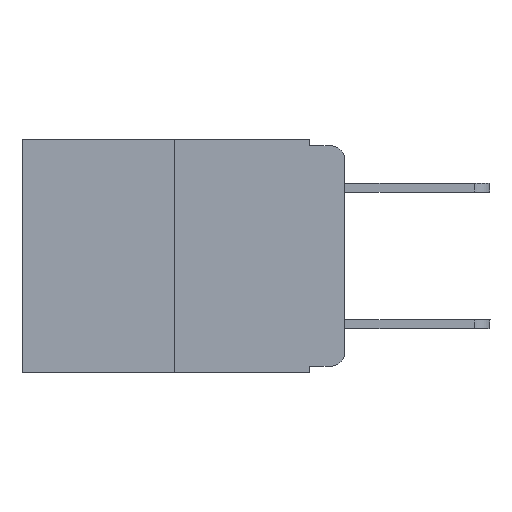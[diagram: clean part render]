
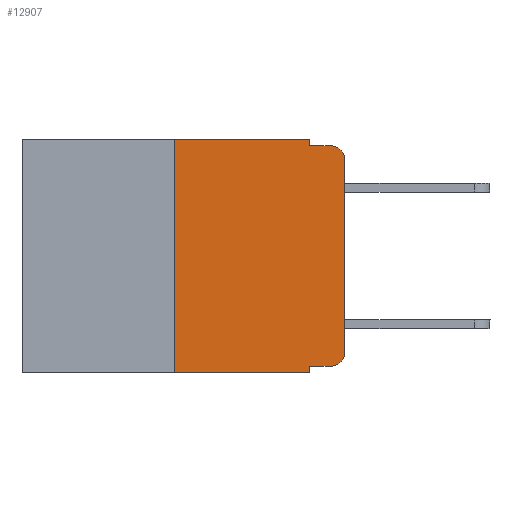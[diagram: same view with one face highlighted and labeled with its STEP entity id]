
A CAD part, left-side view. The second image highlights one B-rep face of the part: STEP entity #12907.
In plain terms, the highlighted planar face has unit normal (-1, 0, 0).
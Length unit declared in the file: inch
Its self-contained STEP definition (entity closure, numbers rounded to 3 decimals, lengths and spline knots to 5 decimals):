
#98 = AXIS2_PLACEMENT_3D ( 'NONE', #14509, #1699, #7501 ) ;
#139 = CARTESIAN_POINT ( 'NONE',  ( 0., 0.25, 0. ) ) ;
#285 = ORIENTED_EDGE ( 'NONE', *, *, #360, .T. ) ;
#360 = EDGE_CURVE ( 'NONE', #15100, #4920, #1604, .T. ) ;
#596 = VERTEX_POINT ( 'NONE', #11716 ) ;
#723 = CARTESIAN_POINT ( 'NONE',  ( 0., 0.051, -0.01 ) ) ;
#1584 = AXIS2_PLACEMENT_3D ( 'NONE', #2844, #2794, #10892 ) ;
#1585 = DIRECTION ( 'NONE',  ( 0., -1., 0. ) ) ;
#1597 = ORIENTED_EDGE ( 'NONE', *, *, #11966, .T. ) ;
#1604 = CIRCLE ( 'NONE', #98, 0.02 ) ;
#1699 = DIRECTION ( 'NONE',  ( -1., 0., 0. ) ) ;
#1790 = LINE ( 'NONE', #139, #7619 ) ;
#2120 = EDGE_CURVE ( 'NONE', #596, #11708, #8279, .T. ) ;
#2179 = CARTESIAN_POINT ( 'NONE',  ( 0., 0.051, 0. ) ) ;
#2493 = DIRECTION ( 'NONE',  ( 0., 0., 1. ) ) ;
#2783 = CARTESIAN_POINT ( 'NONE',  ( 0., 0.25, -0.343 ) ) ;
#2794 = DIRECTION ( 'NONE',  ( 1., 0., 0. ) ) ;
#2844 = CARTESIAN_POINT ( 'NONE',  ( 0., 0.473, 0. ) ) ;
#3056 = CARTESIAN_POINT ( 'NONE',  ( 0., 0.051, 0. ) ) ;
#3266 = VECTOR ( 'NONE', #13097, 39.37008 ) ;
#3449 = ORIENTED_EDGE ( 'NONE', *, *, #2120, .T. ) ;
#4105 = VECTOR ( 'NONE', #1585, 39.37008 ) ;
#4127 = DIRECTION ( 'NONE',  ( 0., -1., 0. ) ) ;
#4250 = VERTEX_POINT ( 'NONE', #3056 ) ;
#4324 = CARTESIAN_POINT ( 'NONE',  ( 0., 0.051, -0.01 ) ) ;
#4416 = ORIENTED_EDGE ( 'NONE', *, *, #10406, .F. ) ;
#4563 = CIRCLE ( 'NONE', #10289, 0.02 ) ;
#4698 = EDGE_LOOP ( 'NONE', ( #13879, #285, #4416, #14814, #10746, #13309, #5383, #13770, #3449, #1597 ) ) ;
#4703 = LINE ( 'NONE', #9688, #3266 ) ;
#4901 = EDGE_CURVE ( 'NONE', #13058, #15100, #7156, .T. ) ;
#4920 = VERTEX_POINT ( 'NONE', #5144 ) ;
#5144 = CARTESIAN_POINT ( 'NONE',  ( 0., 0.02, -0.01 ) ) ;
#5383 = ORIENTED_EDGE ( 'NONE', *, *, #6700, .T. ) ;
#5666 = LINE ( 'NONE', #6740, #9860 ) ;
#5711 = EDGE_CURVE ( 'NONE', #596, #8923, #9313, .T. ) ;
#5781 = DIRECTION ( 'NONE',  ( 0., 0., -1. ) ) ;
#6079 = EDGE_CURVE ( 'NONE', #14229, #4250, #5666, .T. ) ;
#6168 = CARTESIAN_POINT ( 'NONE',  ( 0., 0.051, -0.333 ) ) ;
#6700 = EDGE_CURVE ( 'NONE', #7402, #8923, #4703, .T. ) ;
#6740 = CARTESIAN_POINT ( 'NONE',  ( 0., 0.473, 0. ) ) ;
#7008 = CARTESIAN_POINT ( 'NONE',  ( 0., 0.051, -0.343 ) ) ;
#7156 = LINE ( 'NONE', #12736, #7344 ) ;
#7344 = VECTOR ( 'NONE', #15099, 39.37008 ) ;
#7402 = VERTEX_POINT ( 'NONE', #2783 ) ;
#7501 = DIRECTION ( 'NONE',  ( 0., 0., -1. ) ) ;
#7575 = CARTESIAN_POINT ( 'NONE',  ( 0., 0., -0.313 ) ) ;
#7619 = VECTOR ( 'NONE', #2493, 39.37008 ) ;
#8142 = CARTESIAN_POINT ( 'NONE',  ( 0., 0.02, -0.313 ) ) ;
#8279 = LINE ( 'NONE', #6168, #4105 ) ;
#8289 = EDGE_CURVE ( 'NONE', #7402, #14229, #1790, .T. ) ;
#8463 = CARTESIAN_POINT ( 'NONE',  ( 0., 0., -0.03 ) ) ;
#8923 = VERTEX_POINT ( 'NONE', #7008 ) ;
#8943 = CARTESIAN_POINT ( 'NONE',  ( 0., 0.051, 0. ) ) ;
#9313 = LINE ( 'NONE', #2179, #11502 ) ;
#9338 = DIRECTION ( 'NONE',  ( -1., 0., 0. ) ) ;
#9688 = CARTESIAN_POINT ( 'NONE',  ( 0., 0.473, -0.343 ) ) ;
#9860 = VECTOR ( 'NONE', #13809, 39.37008 ) ;
#10289 = AXIS2_PLACEMENT_3D ( 'NONE', #8142, #9338, #5781 ) ;
#10377 = EDGE_CURVE ( 'NONE', #4250, #12511, #14118, .T. ) ;
#10406 = EDGE_CURVE ( 'NONE', #12511, #4920, #14669, .T. ) ;
#10746 = ORIENTED_EDGE ( 'NONE', *, *, #6079, .F. ) ;
#10892 = DIRECTION ( 'NONE',  ( 0., 0., -1. ) ) ;
#11144 = DIRECTION ( 'NONE',  ( 0., 0., -1. ) ) ;
#11502 = VECTOR ( 'NONE', #11747, 39.37008 ) ;
#11708 = VERTEX_POINT ( 'NONE', #14368 ) ;
#11716 = CARTESIAN_POINT ( 'NONE',  ( 0., 0.051, -0.333 ) ) ;
#11747 = DIRECTION ( 'NONE',  ( 0., 0., -1. ) ) ;
#11966 = EDGE_CURVE ( 'NONE', #11708, #13058, #4563, .T. ) ;
#12365 = CARTESIAN_POINT ( 'NONE',  ( 0., 0.25, 0. ) ) ;
#12505 = PLANE ( 'NONE',  #1584 ) ;
#12511 = VERTEX_POINT ( 'NONE', #723 ) ;
#12736 = CARTESIAN_POINT ( 'NONE',  ( 0., 0., 0. ) ) ;
#12907 = ADVANCED_FACE ( 'NONE', ( #14951 ), #12505, .F. ) ;
#13058 = VERTEX_POINT ( 'NONE', #7575 ) ;
#13097 = DIRECTION ( 'NONE',  ( 0., -1., 0. ) ) ;
#13214 = VECTOR ( 'NONE', #4127, 39.37008 ) ;
#13309 = ORIENTED_EDGE ( 'NONE', *, *, #8289, .F. ) ;
#13770 = ORIENTED_EDGE ( 'NONE', *, *, #5711, .F. ) ;
#13809 = DIRECTION ( 'NONE',  ( 0., -1., 0. ) ) ;
#13879 = ORIENTED_EDGE ( 'NONE', *, *, #4901, .T. ) ;
#14118 = LINE ( 'NONE', #8943, #14310 ) ;
#14229 = VERTEX_POINT ( 'NONE', #12365 ) ;
#14310 = VECTOR ( 'NONE', #11144, 39.37008 ) ;
#14368 = CARTESIAN_POINT ( 'NONE',  ( 0., 0.02, -0.333 ) ) ;
#14509 = CARTESIAN_POINT ( 'NONE',  ( 0., 0.02, -0.03 ) ) ;
#14669 = LINE ( 'NONE', #4324, #13214 ) ;
#14814 = ORIENTED_EDGE ( 'NONE', *, *, #10377, .F. ) ;
#14951 = FACE_OUTER_BOUND ( 'NONE', #4698, .T. ) ;
#15099 = DIRECTION ( 'NONE',  ( 0., 0., 1. ) ) ;
#15100 = VERTEX_POINT ( 'NONE', #8463 ) ;
